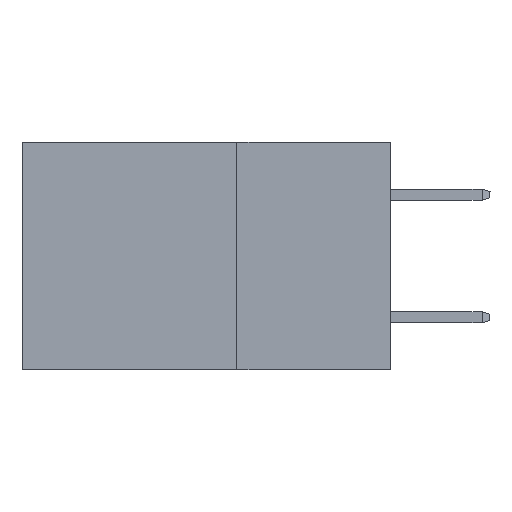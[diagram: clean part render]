
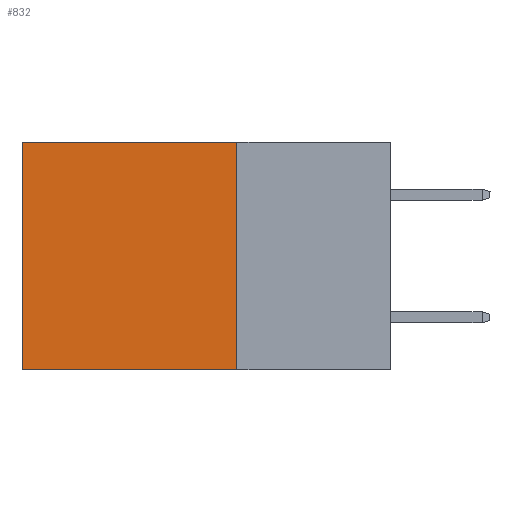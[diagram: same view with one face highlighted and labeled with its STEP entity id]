
A CAD part, left-side view. The second image highlights one B-rep face of the part: STEP entity #832.
In plain terms, the highlighted planar face has unit normal (-1, 0, 0).
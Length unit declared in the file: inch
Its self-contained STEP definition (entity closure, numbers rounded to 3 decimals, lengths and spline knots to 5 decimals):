
#300 = EDGE_LOOP ( 'NONE', ( #4568, #1318, #1822, #7327 ) ) ;
#594 = EDGE_CURVE ( 'NONE', #1420, #8149, #4305, .T. ) ;
#832 = ADVANCED_FACE ( 'NONE', ( #6153 ), #9513, .F. ) ;
#973 = LINE ( 'NONE', #2018, #1556 ) ;
#1041 = VERTEX_POINT ( 'NONE', #5663 ) ;
#1318 = ORIENTED_EDGE ( 'NONE', *, *, #3346, .F. ) ;
#1420 = VERTEX_POINT ( 'NONE', #4728 ) ;
#1556 = VECTOR ( 'NONE', #7224, 39.37008 ) ;
#1622 = EDGE_CURVE ( 'NONE', #8149, #7361, #6366, .T. ) ;
#1738 = CARTESIAN_POINT ( 'NONE',  ( 0.2875, 0.6, -0.37 ) ) ;
#1822 = ORIENTED_EDGE ( 'NONE', *, *, #5210, .F. ) ;
#2018 = CARTESIAN_POINT ( 'NONE',  ( 0.2875, 0.25, 0. ) ) ;
#2324 = VECTOR ( 'NONE', #2333, 39.37008 ) ;
#2333 = DIRECTION ( 'NONE',  ( 0., 1., 0. ) ) ;
#3111 = CARTESIAN_POINT ( 'NONE',  ( 0.2875, 0.6, 0. ) ) ;
#3346 = EDGE_CURVE ( 'NONE', #1041, #7361, #6459, .T. ) ;
#3777 = DIRECTION ( 'NONE',  ( 0., 1., 0. ) ) ;
#3998 = CARTESIAN_POINT ( 'NONE',  ( 0.2875, 0.25, -0.37 ) ) ;
#4085 = AXIS2_PLACEMENT_3D ( 'NONE', #5883, #4348, #6561 ) ;
#4305 = LINE ( 'NONE', #8174, #2324 ) ;
#4348 = DIRECTION ( 'NONE',  ( 1., 0., 0. ) ) ;
#4568 = ORIENTED_EDGE ( 'NONE', *, *, #1622, .T. ) ;
#4728 = CARTESIAN_POINT ( 'NONE',  ( 0.2875, 0.25, 0. ) ) ;
#5210 = EDGE_CURVE ( 'NONE', #1420, #1041, #973, .T. ) ;
#5663 = CARTESIAN_POINT ( 'NONE',  ( 0.2875, 0.25, -0.37 ) ) ;
#5883 = CARTESIAN_POINT ( 'NONE',  ( 0.2875, 0.25, 0. ) ) ;
#6013 = VECTOR ( 'NONE', #8216, 39.37008 ) ;
#6153 = FACE_OUTER_BOUND ( 'NONE', #300, .T. ) ;
#6366 = LINE ( 'NONE', #8114, #6013 ) ;
#6459 = LINE ( 'NONE', #3998, #7042 ) ;
#6561 = DIRECTION ( 'NONE',  ( 0., 0., -1. ) ) ;
#7042 = VECTOR ( 'NONE', #3777, 39.37008 ) ;
#7224 = DIRECTION ( 'NONE',  ( 0., 0., -1. ) ) ;
#7327 = ORIENTED_EDGE ( 'NONE', *, *, #594, .T. ) ;
#7361 = VERTEX_POINT ( 'NONE', #1738 ) ;
#8114 = CARTESIAN_POINT ( 'NONE',  ( 0.2875, 0.6, 0. ) ) ;
#8149 = VERTEX_POINT ( 'NONE', #3111 ) ;
#8174 = CARTESIAN_POINT ( 'NONE',  ( 0.2875, 0.25, 0. ) ) ;
#8216 = DIRECTION ( 'NONE',  ( 0., 0., -1. ) ) ;
#9513 = PLANE ( 'NONE',  #4085 ) ;
